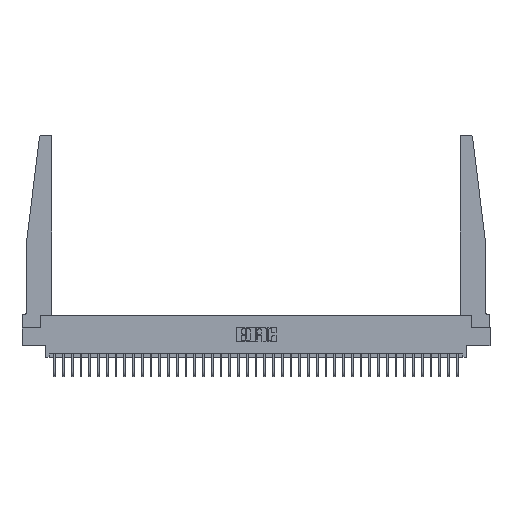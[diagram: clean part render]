
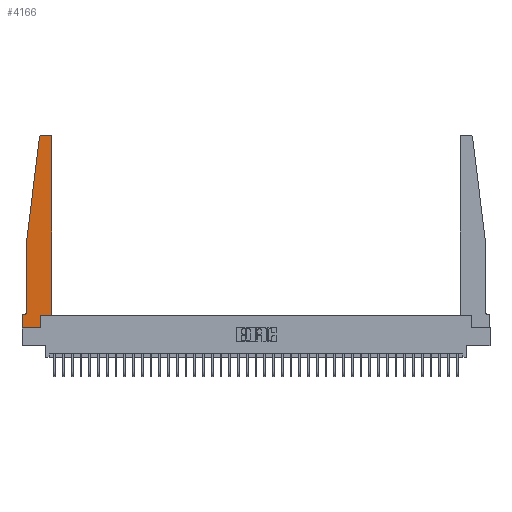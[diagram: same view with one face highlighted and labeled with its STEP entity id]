
A CAD part, top view. The second image highlights one B-rep face of the part: STEP entity #4166.
In plain terms, the highlighted planar face has unit normal (0, 0, 1).
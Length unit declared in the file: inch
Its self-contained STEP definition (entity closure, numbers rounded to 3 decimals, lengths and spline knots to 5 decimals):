
#155 = ORIENTED_EDGE ( 'NONE', *, *, #9861, .T. ) ;
#162 = AXIS2_PLACEMENT_3D ( 'NONE', #24014, #518, #21762 ) ;
#407 = ORIENTED_EDGE ( 'NONE', *, *, #20633, .T. ) ;
#431 = CARTESIAN_POINT ( 'NONE',  ( 0.2605, 0.18, 0.37 ) ) ;
#518 = DIRECTION ( 'NONE',  ( 0., 0., -1. ) ) ;
#600 = VECTOR ( 'NONE', #32740, 39.37008 ) ;
#732 = LINE ( 'NONE', #8084, #22487 ) ;
#970 = AXIS2_PLACEMENT_3D ( 'NONE', #1366, #8879, #27415 ) ;
#1366 = CARTESIAN_POINT ( 'NONE',  ( 0.395, 2.72, 0.37 ) ) ;
#1723 = CARTESIAN_POINT ( 'NONE',  ( 0., 0., 0.37 ) ) ;
#1728 = DIRECTION ( 'NONE',  ( 0., -1., 0. ) ) ;
#1758 = VERTEX_POINT ( 'NONE', #28350 ) ;
#1918 = CARTESIAN_POINT ( 'NONE',  ( 0.27653, 2.72, 0.37 ) ) ;
#2425 = CARTESIAN_POINT ( 'NONE',  ( 0.065, 1.25, 0.37 ) ) ;
#3151 = DIRECTION ( 'NONE',  ( 1., 0., 0. ) ) ;
#3601 = VERTEX_POINT ( 'NONE', #24318 ) ;
#3606 = ORIENTED_EDGE ( 'NONE', *, *, #13953, .T. ) ;
#3872 = VERTEX_POINT ( 'NONE', #14139 ) ;
#3988 = ORIENTED_EDGE ( 'NONE', *, *, #20309, .T. ) ;
#4166 = ADVANCED_FACE ( 'NONE', ( #4878 ), #24950, .T. ) ;
#4214 = DIRECTION ( 'NONE',  ( 1., 0., 0. ) ) ;
#4356 = VERTEX_POINT ( 'NONE', #24063 ) ;
#4878 = FACE_OUTER_BOUND ( 'NONE', #29217, .T. ) ;
#5172 = ORIENTED_EDGE ( 'NONE', *, *, #31496, .T. ) ;
#6600 = CARTESIAN_POINT ( 'NONE',  ( 0.065, 0.1875, 0.37 ) ) ;
#6691 = CARTESIAN_POINT ( 'NONE',  ( 0.24675, 2.72367, 0.37 ) ) ;
#6772 = CARTESIAN_POINT ( 'NONE',  ( 0., 0.1875, 0.37 ) ) ;
#7392 = LINE ( 'NONE', #12877, #8976 ) ;
#7546 = ORIENTED_EDGE ( 'NONE', *, *, #21040, .T. ) ;
#8084 = CARTESIAN_POINT ( 'NONE',  ( 0.065, 1.25, 0.37 ) ) ;
#8879 = DIRECTION ( 'NONE',  ( 0., 0., 1. ) ) ;
#8976 = VECTOR ( 'NONE', #33476, 39.37008 ) ;
#9041 = CARTESIAN_POINT ( 'NONE',  ( 0.25, 2.75, 0.37 ) ) ;
#9062 = VERTEX_POINT ( 'NONE', #1723 ) ;
#9431 = CARTESIAN_POINT ( 'NONE',  ( 0., 0., 0.37 ) ) ;
#9861 = EDGE_CURVE ( 'NONE', #31013, #31250, #13954, .T. ) ;
#10849 = CIRCLE ( 'NONE', #970, 0.03 ) ;
#11797 = CARTESIAN_POINT ( 'NONE',  ( 0.425, 0.18, 0.37 ) ) ;
#12877 = CARTESIAN_POINT ( 'NONE',  ( 0.425, 0.18, 0.37 ) ) ;
#13101 = VERTEX_POINT ( 'NONE', #32543 ) ;
#13615 = LINE ( 'NONE', #431, #21943 ) ;
#13953 = EDGE_CURVE ( 'NONE', #13101, #23092, #10849, .T. ) ;
#13954 = LINE ( 'NONE', #24406, #14832 ) ;
#13980 = VERTEX_POINT ( 'NONE', #32413 ) ;
#14139 = CARTESIAN_POINT ( 'NONE',  ( 0.015, 0.1875, 0.37 ) ) ;
#14585 = LINE ( 'NONE', #9431, #29653 ) ;
#14832 = VECTOR ( 'NONE', #24557, 39.37008 ) ;
#14926 = CIRCLE ( 'NONE', #162, 0.05 ) ;
#15241 = DIRECTION ( 'NONE',  ( 0., 0., 1. ) ) ;
#16459 = VERTEX_POINT ( 'NONE', #24713 ) ;
#16498 = CARTESIAN_POINT ( 'NONE',  ( 0., 0.1875, 0.37 ) ) ;
#16564 = EDGE_CURVE ( 'NONE', #4356, #13101, #7392, .T. ) ;
#16758 = CARTESIAN_POINT ( 'NONE',  ( 0.395, 2.75, 0.37 ) ) ;
#17224 = DIRECTION ( 'NONE',  ( 0., 0., 1. ) ) ;
#17826 = EDGE_CURVE ( 'NONE', #3601, #3872, #14926, .T. ) ;
#18681 = VECTOR ( 'NONE', #32373, 39.37008 ) ;
#18749 = DIRECTION ( 'NONE',  ( 0., -1., 0. ) ) ;
#19506 = ORIENTED_EDGE ( 'NONE', *, *, #20097, .T. ) ;
#19683 = DIRECTION ( 'NONE',  ( -1., 0., 0. ) ) ;
#20097 = EDGE_CURVE ( 'NONE', #16459, #31013, #27425, .T. ) ;
#20309 = EDGE_CURVE ( 'NONE', #13980, #4356, #24483, .T. ) ;
#20633 = EDGE_CURVE ( 'NONE', #1758, #13980, #13615, .T. ) ;
#21040 = EDGE_CURVE ( 'NONE', #31250, #3601, #732, .T. ) ;
#21762 = DIRECTION ( 'NONE',  ( -1., 0., 0. ) ) ;
#21943 = VECTOR ( 'NONE', #27185, 39.37008 ) ;
#22095 = LINE ( 'NONE', #9041, #27648 ) ;
#22487 = VECTOR ( 'NONE', #18749, 39.37008 ) ;
#23092 = VERTEX_POINT ( 'NONE', #16758 ) ;
#23557 = LINE ( 'NONE', #26147, #30160 ) ;
#24014 = CARTESIAN_POINT ( 'NONE',  ( 0.015, 0.2375, 0.37 ) ) ;
#24063 = CARTESIAN_POINT ( 'NONE',  ( 0.425, 0.18, 0.37 ) ) ;
#24234 = ORIENTED_EDGE ( 'NONE', *, *, #32992, .T. ) ;
#24318 = CARTESIAN_POINT ( 'NONE',  ( 0.065, 0.2375, 0.37 ) ) ;
#24406 = CARTESIAN_POINT ( 'NONE',  ( 0.065, 1.25, 0.37 ) ) ;
#24483 = LINE ( 'NONE', #11797, #600 ) ;
#24557 = DIRECTION ( 'NONE',  ( -0.122, -0.992, 0. ) ) ;
#24713 = CARTESIAN_POINT ( 'NONE',  ( 0.27653, 2.75, 0.37 ) ) ;
#24950 = PLANE ( 'NONE',  #26349 ) ;
#24972 = LINE ( 'NONE', #6600, #18681 ) ;
#25563 = DIRECTION ( 'NONE',  ( 1., 0., 0. ) ) ;
#26147 = CARTESIAN_POINT ( 'NONE',  ( 0., 0., 0.37 ) ) ;
#26349 = AXIS2_PLACEMENT_3D ( 'NONE', #6772, #17224, #4214 ) ;
#27185 = DIRECTION ( 'NONE',  ( 0., 1., 0. ) ) ;
#27415 = DIRECTION ( 'NONE',  ( 1., 0., 0. ) ) ;
#27425 = CIRCLE ( 'NONE', #31838, 0.03 ) ;
#27590 = EDGE_CURVE ( 'NONE', #30506, #9062, #14585, .T. ) ;
#27648 = VECTOR ( 'NONE', #19683, 39.37008 ) ;
#28350 = CARTESIAN_POINT ( 'NONE',  ( 0.2605, 0., 0.37 ) ) ;
#28729 = ORIENTED_EDGE ( 'NONE', *, *, #27590, .T. ) ;
#29217 = EDGE_LOOP ( 'NONE', ( #5172, #19506, #155, #7546, #32907, #24234, #28729, #32722, #407, #3988, #31288, #3606 ) ) ;
#29653 = VECTOR ( 'NONE', #1728, 39.37008 ) ;
#30160 = VECTOR ( 'NONE', #3151, 39.37008 ) ;
#30506 = VERTEX_POINT ( 'NONE', #16498 ) ;
#31013 = VERTEX_POINT ( 'NONE', #6691 ) ;
#31250 = VERTEX_POINT ( 'NONE', #2425 ) ;
#31288 = ORIENTED_EDGE ( 'NONE', *, *, #16564, .T. ) ;
#31496 = EDGE_CURVE ( 'NONE', #23092, #16459, #22095, .T. ) ;
#31838 = AXIS2_PLACEMENT_3D ( 'NONE', #1918, #15241, #25563 ) ;
#32373 = DIRECTION ( 'NONE',  ( -1., 0., 0. ) ) ;
#32413 = CARTESIAN_POINT ( 'NONE',  ( 0.2605, 0.18, 0.37 ) ) ;
#32543 = CARTESIAN_POINT ( 'NONE',  ( 0.425, 2.72, 0.37 ) ) ;
#32722 = ORIENTED_EDGE ( 'NONE', *, *, #33677, .T. ) ;
#32740 = DIRECTION ( 'NONE',  ( 1., 0., 0. ) ) ;
#32907 = ORIENTED_EDGE ( 'NONE', *, *, #17826, .T. ) ;
#32992 = EDGE_CURVE ( 'NONE', #3872, #30506, #24972, .T. ) ;
#33476 = DIRECTION ( 'NONE',  ( 0., 1., 0. ) ) ;
#33677 = EDGE_CURVE ( 'NONE', #9062, #1758, #23557, .T. ) ;
